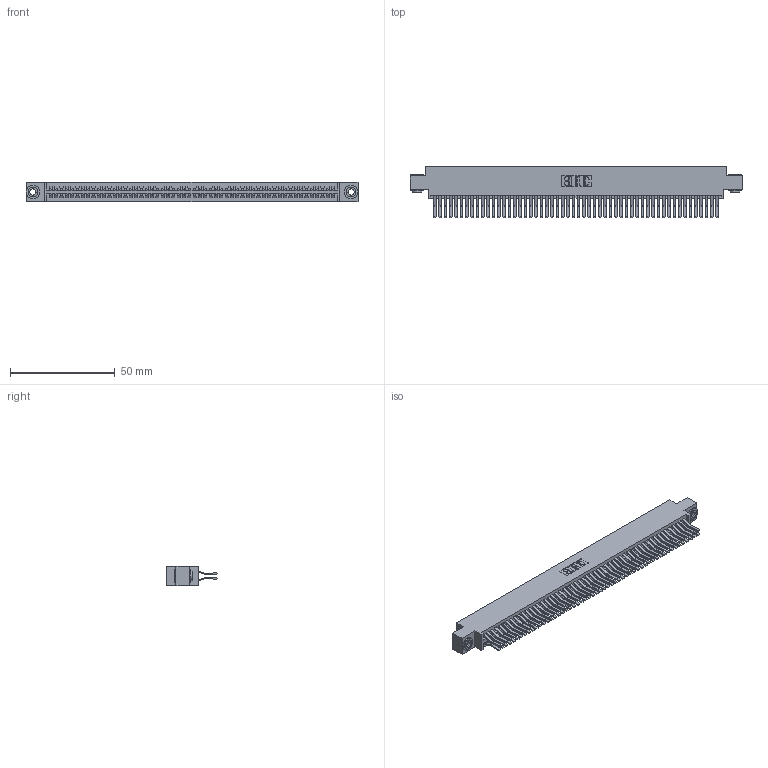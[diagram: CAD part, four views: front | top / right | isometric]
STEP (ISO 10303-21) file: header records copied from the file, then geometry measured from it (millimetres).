
FILE_DESCRIPTION (( 'STEP AP203' ), '1' );
FILE_NAME ('345-108-560-803.STEP', '2019-11-04T15:14:56', ( '' ), ( '' ), 'SwSTEP 2.0', 'SolidWorks 2016', '' );
FILE_SCHEMA (( 'CONFIG_CONTROL_DESIGN' ));
Length unit declared in the file: inch
Products named in the file (4): 345-108-560-803; 345-292-001_560 Tail; 345 Part_0.170 Offset - 0.156 Dia-TH; 345-250-002_345-250-002-102
Assembly tree (111 placements, depth 2):
  345-108-560-803
    345 Part_0.170 Offset - 0.156 Dia-TH
    345-292-001_560 Tail  x108
    345-250-002_345-250-002-102  x2
Bounding box: 158.37 x 24.45 x 9.4 mm (x, y, z)
Volume: 16109.4 mm3; surface area: 26213.9 mm2
Topology: 111 solids, 111 shells, 5784 faces, 17169 edges, 11298 vertices
Faces by surface type: plane 3658, cylinder 2118, cone 8
Entity records: 41624 total; most frequent: CARTESIAN_POINT 6943, ORIENTED_EDGE 6870, DIRECTION 6141, EDGE_CURVE 3435, LINE 3059, VECTOR 3059, VERTEX_POINT 2286, AXIS2_PLACEMENT_3D 1541
